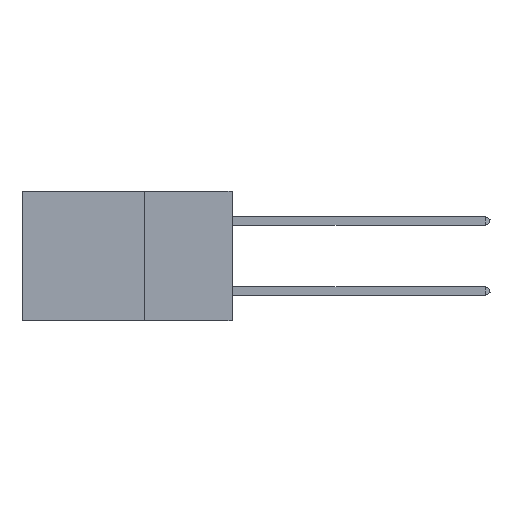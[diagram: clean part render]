
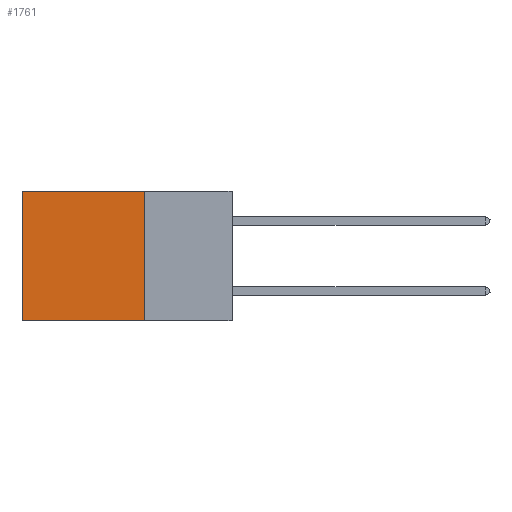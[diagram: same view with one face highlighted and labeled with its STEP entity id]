
A CAD part, left-side view. The second image highlights one B-rep face of the part: STEP entity #1761.
In plain terms, the highlighted planar face has unit normal (-1, 0, 0).
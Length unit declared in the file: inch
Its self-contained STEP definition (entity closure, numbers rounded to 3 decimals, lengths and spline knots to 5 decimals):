
#1761 = ADVANCED_FACE ( 'NONE', ( #16790 ), #25140, .F. ) ;
#1934 = DIRECTION ( 'NONE',  ( 0., 0., -1. ) ) ;
#2434 = EDGE_CURVE ( 'NONE', #34837, #11310, #6164, .T. ) ;
#3814 = CARTESIAN_POINT ( 'NONE',  ( 0.2875, 0.25, 0. ) ) ;
#3994 = CARTESIAN_POINT ( 'NONE',  ( 0.2875, 0.6, 0. ) ) ;
#5691 = VECTOR ( 'NONE', #7654, 39.37008 ) ;
#6164 = LINE ( 'NONE', #16849, #5691 ) ;
#7433 = VECTOR ( 'NONE', #15374, 39.37008 ) ;
#7654 = DIRECTION ( 'NONE',  ( 0., 0., -1. ) ) ;
#11310 = VERTEX_POINT ( 'NONE', #25793 ) ;
#12284 = VERTEX_POINT ( 'NONE', #3814 ) ;
#13652 = EDGE_CURVE ( 'NONE', #12284, #22761, #27106, .T. ) ;
#14789 = AXIS2_PLACEMENT_3D ( 'NONE', #16435, #36782, #1934 ) ;
#15374 = DIRECTION ( 'NONE',  ( 0., 0., -1. ) ) ;
#16173 = ORIENTED_EDGE ( 'NONE', *, *, #2434, .T. ) ;
#16435 = CARTESIAN_POINT ( 'NONE',  ( 0.2875, 0.25, 0. ) ) ;
#16743 = LINE ( 'NONE', #30500, #17665 ) ;
#16790 = FACE_OUTER_BOUND ( 'NONE', #29674, .T. ) ;
#16849 = CARTESIAN_POINT ( 'NONE',  ( 0.2875, 0.6, 0. ) ) ;
#17665 = VECTOR ( 'NONE', #36647, 39.37008 ) ;
#18706 = CARTESIAN_POINT ( 'NONE',  ( 0.2875, 0.25, 0. ) ) ;
#22433 = ORIENTED_EDGE ( 'NONE', *, *, #13652, .F. ) ;
#22761 = VERTEX_POINT ( 'NONE', #35353 ) ;
#23206 = VECTOR ( 'NONE', #27016, 39.37008 ) ;
#25140 = PLANE ( 'NONE',  #14789 ) ;
#25571 = LINE ( 'NONE', #35712, #23206 ) ;
#25793 = CARTESIAN_POINT ( 'NONE',  ( 0.2875, 0.6, -0.37 ) ) ;
#27016 = DIRECTION ( 'NONE',  ( 0., 1., 0. ) ) ;
#27106 = LINE ( 'NONE', #18706, #7433 ) ;
#29674 = EDGE_LOOP ( 'NONE', ( #16173, #29820, #22433, #35155 ) ) ;
#29820 = ORIENTED_EDGE ( 'NONE', *, *, #32500, .F. ) ;
#30500 = CARTESIAN_POINT ( 'NONE',  ( 0.2875, 0.25, 0. ) ) ;
#32500 = EDGE_CURVE ( 'NONE', #22761, #11310, #25571, .T. ) ;
#34003 = EDGE_CURVE ( 'NONE', #12284, #34837, #16743, .T. ) ;
#34837 = VERTEX_POINT ( 'NONE', #3994 ) ;
#35155 = ORIENTED_EDGE ( 'NONE', *, *, #34003, .T. ) ;
#35353 = CARTESIAN_POINT ( 'NONE',  ( 0.2875, 0.25, -0.37 ) ) ;
#35712 = CARTESIAN_POINT ( 'NONE',  ( 0.2875, 0.25, -0.37 ) ) ;
#36647 = DIRECTION ( 'NONE',  ( 0., 1., 0. ) ) ;
#36782 = DIRECTION ( 'NONE',  ( 1., 0., 0. ) ) ;
